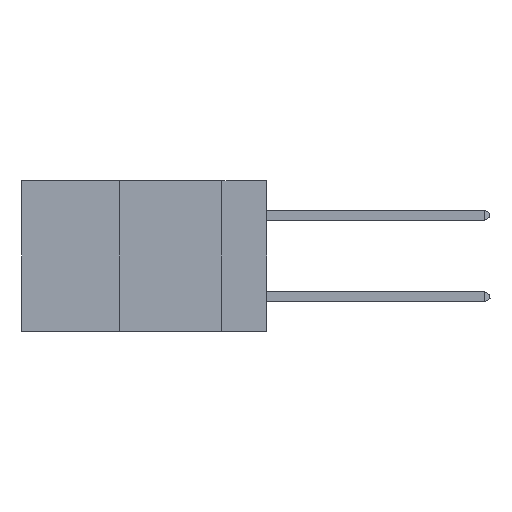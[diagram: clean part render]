
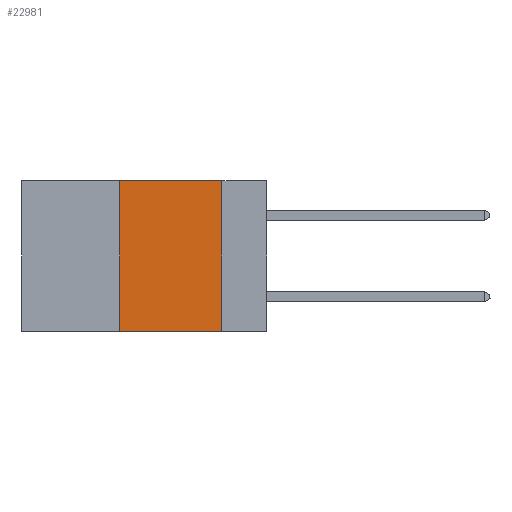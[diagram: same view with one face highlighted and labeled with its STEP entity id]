
A CAD part, left-side view. The second image highlights one B-rep face of the part: STEP entity #22981.
In plain terms, the highlighted planar face has unit normal (-1, 0, 0).
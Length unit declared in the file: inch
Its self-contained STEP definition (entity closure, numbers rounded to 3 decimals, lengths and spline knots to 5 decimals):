
#289 = VECTOR ( 'NONE', #18205, 39.37008 ) ;
#806 = CARTESIAN_POINT ( 'NONE',  ( 0., 0.11, 0. ) ) ;
#1648 = DIRECTION ( 'NONE',  ( 1., 0., 0. ) ) ;
#1717 = EDGE_CURVE ( 'NONE', #10294, #7778, #12527, .T. ) ;
#2100 = ORIENTED_EDGE ( 'NONE', *, *, #1717, .T. ) ;
#2505 = VERTEX_POINT ( 'NONE', #806 ) ;
#2719 = FACE_OUTER_BOUND ( 'NONE', #12148, .T. ) ;
#3135 = DIRECTION ( 'NONE',  ( 0., 0., -1. ) ) ;
#3633 = CARTESIAN_POINT ( 'NONE',  ( 0., 0.36, 0. ) ) ;
#5985 = ORIENTED_EDGE ( 'NONE', *, *, #6978, .F. ) ;
#5995 = VECTOR ( 'NONE', #13211, 39.37008 ) ;
#6477 = AXIS2_PLACEMENT_3D ( 'NONE', #14242, #1648, #3135 ) ;
#6978 = EDGE_CURVE ( 'NONE', #2505, #7778, #21732, .T. ) ;
#7192 = VECTOR ( 'NONE', #17221, 39.37008 ) ;
#7778 = VERTEX_POINT ( 'NONE', #16313 ) ;
#9462 = VECTOR ( 'NONE', #13742, 39.37008 ) ;
#10294 = VERTEX_POINT ( 'NONE', #18628 ) ;
#11944 = CARTESIAN_POINT ( 'NONE',  ( 0., 0.6, -0.37 ) ) ;
#12148 = EDGE_LOOP ( 'NONE', ( #5985, #22973, #14490, #2100 ) ) ;
#12527 = LINE ( 'NONE', #11944, #9462 ) ;
#13211 = DIRECTION ( 'NONE',  ( 0., -1., 0. ) ) ;
#13676 = CARTESIAN_POINT ( 'NONE',  ( 0., 0.36, 0. ) ) ;
#13742 = DIRECTION ( 'NONE',  ( 0., -1., 0. ) ) ;
#14242 = CARTESIAN_POINT ( 'NONE',  ( 0., 0.6, 0. ) ) ;
#14325 = CARTESIAN_POINT ( 'NONE',  ( 0., 0.11, 0. ) ) ;
#14490 = ORIENTED_EDGE ( 'NONE', *, *, #22918, .F. ) ;
#16313 = CARTESIAN_POINT ( 'NONE',  ( 0., 0.11, -0.37 ) ) ;
#17221 = DIRECTION ( 'NONE',  ( 0., 0., 1. ) ) ;
#17445 = VERTEX_POINT ( 'NONE', #3633 ) ;
#17839 = EDGE_CURVE ( 'NONE', #17445, #2505, #18113, .T. ) ;
#18113 = LINE ( 'NONE', #20455, #5995 ) ;
#18205 = DIRECTION ( 'NONE',  ( 0., 0., -1. ) ) ;
#18520 = LINE ( 'NONE', #13676, #7192 ) ;
#18628 = CARTESIAN_POINT ( 'NONE',  ( 0., 0.36, -0.37 ) ) ;
#20455 = CARTESIAN_POINT ( 'NONE',  ( 0., 0.6, 0. ) ) ;
#21732 = LINE ( 'NONE', #14325, #289 ) ;
#22918 = EDGE_CURVE ( 'NONE', #10294, #17445, #18520, .T. ) ;
#22973 = ORIENTED_EDGE ( 'NONE', *, *, #17839, .F. ) ;
#22981 = ADVANCED_FACE ( 'NONE', ( #2719 ), #23246, .F. ) ;
#23246 = PLANE ( 'NONE',  #6477 ) ;
